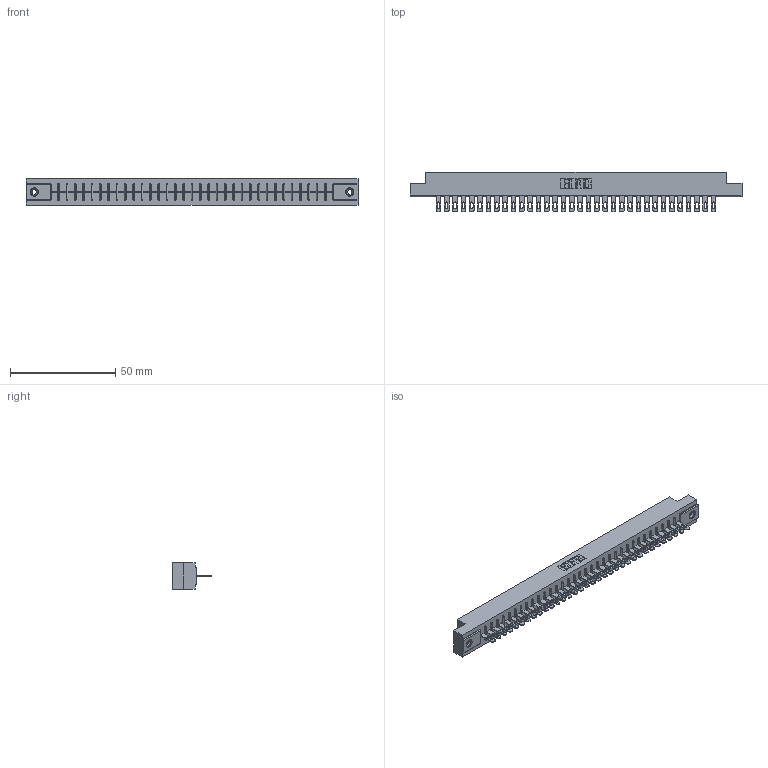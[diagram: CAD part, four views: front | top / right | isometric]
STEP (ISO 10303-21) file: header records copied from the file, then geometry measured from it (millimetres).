
FILE_DESCRIPTION (( 'STEP AP203' ), '1' );
FILE_NAME ('306-034-400-108.STEP', '2020-09-22T03:10:41', ( '' ), ( '' ), 'SwSTEP 2.0', 'SolidWorks 2020', '' );
FILE_SCHEMA (( 'CONFIG_CONTROL_DESIGN' ));
Length unit declared in the file: inch
Products named in the file (4): 306-290-001_100; 306 Part_.156 Dia; 306-034-400-108; 345-250-001_345-250-003-102
Assembly tree (37 placements, depth 2):
  306-034-400-108
    306 Part_.156 Dia
    306-290-001_100  x34
    345-250-001_345-250-003-102  x2
Bounding box: 157.73 x 18.87 x 12.7 mm (x, y, z)
Volume: 17471.6 mm3; surface area: 18472.3 mm2
Topology: 37 solids, 37 shells, 2760 faces, 7762 edges, 4984 vertices
Faces by surface type: plane 1800, cylinder 808, sphere 136, cone 12, torus 4
Entity records: 34092 total; most frequent: CARTESIAN_POINT 5704, ORIENTED_EDGE 5648, DIRECTION 5634, EDGE_CURVE 2824, VECTOR 2202, LINE 2202, VERTEX_POINT 1786, AXIS2_PLACEMENT_3D 1716
